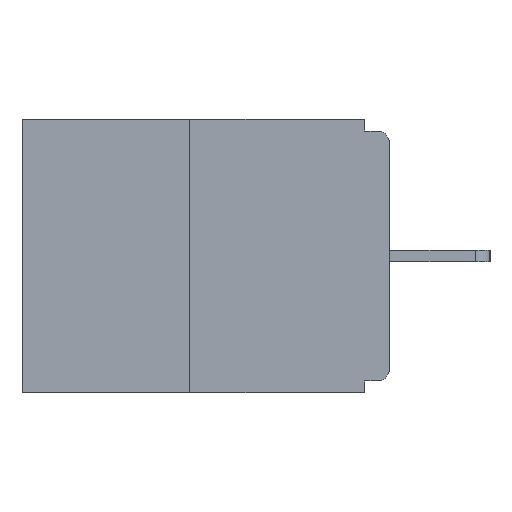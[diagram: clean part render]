
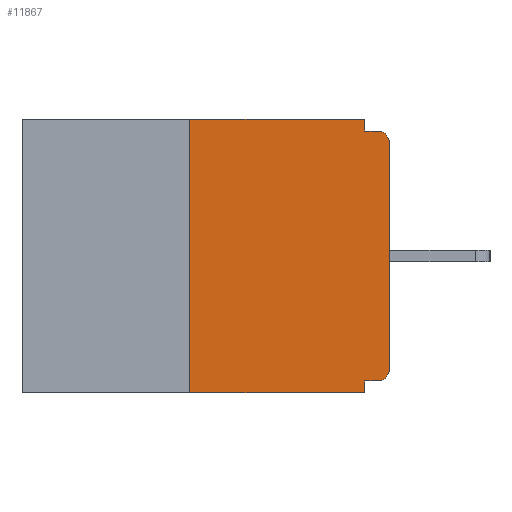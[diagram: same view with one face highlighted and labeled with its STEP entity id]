
A CAD part, left-side view. The second image highlights one B-rep face of the part: STEP entity #11867.
In plain terms, the highlighted planar face has unit normal (-1, 0, 0).
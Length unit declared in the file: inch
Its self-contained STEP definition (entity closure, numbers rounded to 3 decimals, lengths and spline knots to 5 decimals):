
#16 = ORIENTED_EDGE ( 'NONE', *, *, #14024, .F. ) ;
#269 = LINE ( 'NONE', #4248, #17180 ) ;
#992 = LINE ( 'NONE', #17362, #14474 ) ;
#1138 = VECTOR ( 'NONE', #6751, 39.37008 ) ;
#1321 = CARTESIAN_POINT ( 'NONE',  ( 0., 0.46, 0. ) ) ;
#1623 = EDGE_CURVE ( 'NONE', #6945, #16428, #992, .T. ) ;
#1637 = PLANE ( 'NONE',  #5420 ) ;
#1753 = ORIENTED_EDGE ( 'NONE', *, *, #6870, .T. ) ;
#2546 = EDGE_LOOP ( 'NONE', ( #4379, #11712, #11820, #2655, #2962, #4917, #1753, #10169, #7123, #16 ) ) ;
#2655 = ORIENTED_EDGE ( 'NONE', *, *, #14216, .F. ) ;
#2871 = VECTOR ( 'NONE', #15007, 39.37008 ) ;
#2962 = ORIENTED_EDGE ( 'NONE', *, *, #16148, .F. ) ;
#3496 = LINE ( 'NONE', #14549, #4593 ) ;
#3731 = CARTESIAN_POINT ( 'NONE',  ( 0., 0.25, -0.343 ) ) ;
#3950 = DIRECTION ( 'NONE',  ( 0., 1., 0. ) ) ;
#4037 = LINE ( 'NONE', #12370, #10108 ) ;
#4248 = CARTESIAN_POINT ( 'NONE',  ( 0., 0., -0.015 ) ) ;
#4379 = ORIENTED_EDGE ( 'NONE', *, *, #16115, .F. ) ;
#4546 = VECTOR ( 'NONE', #12059, 39.37008 ) ;
#4593 = VECTOR ( 'NONE', #8852, 39.37008 ) ;
#4619 = FACE_OUTER_BOUND ( 'NONE', #2546, .T. ) ;
#4740 = CARTESIAN_POINT ( 'NONE',  ( 0., 0.015, -0.328 ) ) ;
#4917 = ORIENTED_EDGE ( 'NONE', *, *, #11400, .T. ) ;
#5420 = AXIS2_PLACEMENT_3D ( 'NONE', #8793, #12954, #7519 ) ;
#5711 = CARTESIAN_POINT ( 'NONE',  ( 0., 0.015, -0.015 ) ) ;
#5713 = DIRECTION ( 'NONE',  ( -1., 0., 0. ) ) ;
#5865 = DIRECTION ( 'NONE',  ( 0., -1., 0. ) ) ;
#6505 = DIRECTION ( 'NONE',  ( 0., 0., 1. ) ) ;
#6570 = LINE ( 'NONE', #9560, #1138 ) ;
#6751 = DIRECTION ( 'NONE',  ( 0., 0., -1. ) ) ;
#6837 = CIRCLE ( 'NONE', #16945, 0.015 ) ;
#6870 = EDGE_CURVE ( 'NONE', #12451, #9468, #9614, .T. ) ;
#6945 = VERTEX_POINT ( 'NONE', #3731 ) ;
#7123 = ORIENTED_EDGE ( 'NONE', *, *, #8962, .F. ) ;
#7519 = DIRECTION ( 'NONE',  ( 0., 0., -1. ) ) ;
#8128 = CARTESIAN_POINT ( 'NONE',  ( 0., 0.015, -0.03 ) ) ;
#8703 = CARTESIAN_POINT ( 'NONE',  ( 0., 0.031, -0.015 ) ) ;
#8793 = CARTESIAN_POINT ( 'NONE',  ( 0., 0.46, 0. ) ) ;
#8852 = DIRECTION ( 'NONE',  ( 0., 0., -1. ) ) ;
#8907 = AXIS2_PLACEMENT_3D ( 'NONE', #8128, #13662, #13570 ) ;
#8911 = VERTEX_POINT ( 'NONE', #12417 ) ;
#8962 = EDGE_CURVE ( 'NONE', #11845, #14765, #269, .T. ) ;
#9468 = VERTEX_POINT ( 'NONE', #16890 ) ;
#9560 = CARTESIAN_POINT ( 'NONE',  ( 0., 0.031, -0.343 ) ) ;
#9614 = LINE ( 'NONE', #10898, #13182 ) ;
#9949 = VERTEX_POINT ( 'NONE', #14525 ) ;
#10108 = VECTOR ( 'NONE', #3950, 39.37008 ) ;
#10169 = ORIENTED_EDGE ( 'NONE', *, *, #12542, .T. ) ;
#10343 = CARTESIAN_POINT ( 'NONE',  ( 0., 0.46, -0.343 ) ) ;
#10898 = CARTESIAN_POINT ( 'NONE',  ( 0., 0., 0. ) ) ;
#11400 = EDGE_CURVE ( 'NONE', #14410, #12451, #6837, .T. ) ;
#11529 = VERTEX_POINT ( 'NONE', #15691 ) ;
#11572 = EDGE_CURVE ( 'NONE', #6945, #9949, #17209, .T. ) ;
#11712 = ORIENTED_EDGE ( 'NONE', *, *, #1623, .F. ) ;
#11802 = CARTESIAN_POINT ( 'NONE',  ( 0., 0.25, 0. ) ) ;
#11820 = ORIENTED_EDGE ( 'NONE', *, *, #11572, .T. ) ;
#11845 = VERTEX_POINT ( 'NONE', #8703 ) ;
#11867 = ADVANCED_FACE ( 'NONE', ( #4619 ), #1637, .F. ) ;
#11974 = DIRECTION ( 'NONE',  ( 0., 0., 1. ) ) ;
#12059 = DIRECTION ( 'NONE',  ( 0., -1., 0. ) ) ;
#12370 = CARTESIAN_POINT ( 'NONE',  ( 0., 0., -0.328 ) ) ;
#12417 = CARTESIAN_POINT ( 'NONE',  ( 0., 0.031, -0.328 ) ) ;
#12451 = VERTEX_POINT ( 'NONE', #13117 ) ;
#12542 = EDGE_CURVE ( 'NONE', #9468, #14765, #14701, .T. ) ;
#12616 = CARTESIAN_POINT ( 'NONE',  ( 0., 0.015, -0.313 ) ) ;
#12954 = DIRECTION ( 'NONE',  ( 1., 0., 0. ) ) ;
#13117 = CARTESIAN_POINT ( 'NONE',  ( 0., 0., -0.313 ) ) ;
#13182 = VECTOR ( 'NONE', #11974, 39.37008 ) ;
#13570 = DIRECTION ( 'NONE',  ( 0., 0., -1. ) ) ;
#13662 = DIRECTION ( 'NONE',  ( -1., 0., 0. ) ) ;
#14024 = EDGE_CURVE ( 'NONE', #11529, #11845, #3496, .T. ) ;
#14216 = EDGE_CURVE ( 'NONE', #8911, #9949, #6570, .T. ) ;
#14410 = VERTEX_POINT ( 'NONE', #4740 ) ;
#14474 = VECTOR ( 'NONE', #6505, 39.37008 ) ;
#14525 = CARTESIAN_POINT ( 'NONE',  ( 0., 0.031, -0.343 ) ) ;
#14549 = CARTESIAN_POINT ( 'NONE',  ( 0., 0.031, 0. ) ) ;
#14701 = CIRCLE ( 'NONE', #8907, 0.015 ) ;
#14765 = VERTEX_POINT ( 'NONE', #5711 ) ;
#15007 = DIRECTION ( 'NONE',  ( 0., -1., 0. ) ) ;
#15096 = LINE ( 'NONE', #1321, #2871 ) ;
#15691 = CARTESIAN_POINT ( 'NONE',  ( 0., 0.031, 0. ) ) ;
#16115 = EDGE_CURVE ( 'NONE', #16428, #11529, #15096, .T. ) ;
#16148 = EDGE_CURVE ( 'NONE', #14410, #8911, #4037, .T. ) ;
#16421 = DIRECTION ( 'NONE',  ( 0., 0., -1. ) ) ;
#16428 = VERTEX_POINT ( 'NONE', #11802 ) ;
#16890 = CARTESIAN_POINT ( 'NONE',  ( 0., 0., -0.03 ) ) ;
#16945 = AXIS2_PLACEMENT_3D ( 'NONE', #12616, #5713, #16421 ) ;
#17180 = VECTOR ( 'NONE', #5865, 39.37008 ) ;
#17209 = LINE ( 'NONE', #10343, #4546 ) ;
#17362 = CARTESIAN_POINT ( 'NONE',  ( 0., 0.25, 0. ) ) ;
